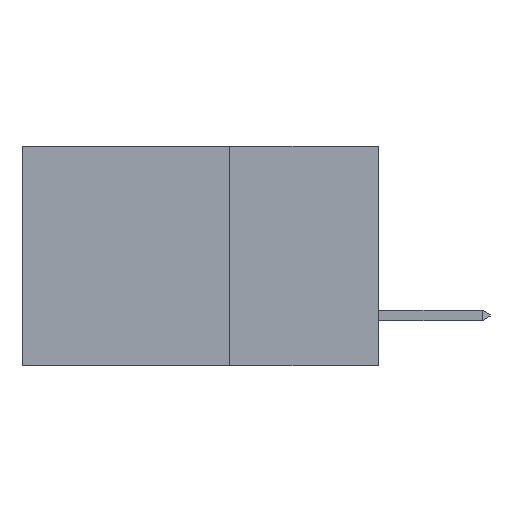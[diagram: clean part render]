
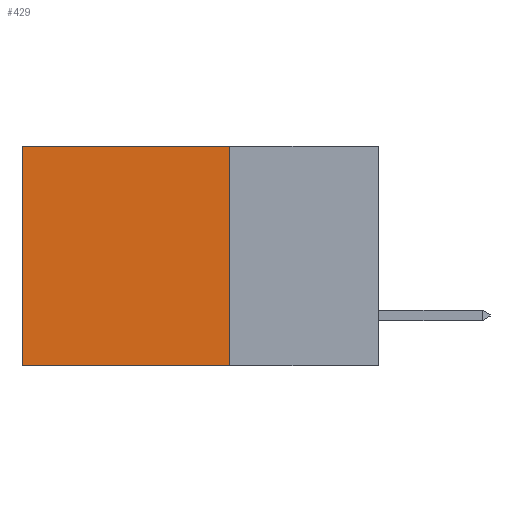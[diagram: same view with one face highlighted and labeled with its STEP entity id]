
A CAD part, left-side view. The second image highlights one B-rep face of the part: STEP entity #429.
In plain terms, the highlighted planar face has unit normal (-1, 0, 0).
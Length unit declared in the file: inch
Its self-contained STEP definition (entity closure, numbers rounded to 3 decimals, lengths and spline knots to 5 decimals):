
#268 = ORIENTED_EDGE ( 'NONE', *, *, #1162, .T. ) ;
#333 = DIRECTION ( 'NONE',  ( 0., 0., -1. ) ) ;
#345 = CARTESIAN_POINT ( 'NONE',  ( 0.2615, 0.6, -0.37 ) ) ;
#382 = CARTESIAN_POINT ( 'NONE',  ( 0.2615, 0.25, -0.37 ) ) ;
#429 = ADVANCED_FACE ( 'NONE', ( #8978 ), #9218, .F. ) ;
#729 = DIRECTION ( 'NONE',  ( 0., 0., -1. ) ) ;
#1162 = EDGE_CURVE ( 'NONE', #4390, #11350, #7078, .T. ) ;
#1446 = EDGE_CURVE ( 'NONE', #10624, #2343, #7065, .T. ) ;
#1938 = ORIENTED_EDGE ( 'NONE', *, *, #1446, .F. ) ;
#2027 = ORIENTED_EDGE ( 'NONE', *, *, #3308, .T. ) ;
#2343 = VERTEX_POINT ( 'NONE', #7645 ) ;
#2366 = LINE ( 'NONE', #345, #7023 ) ;
#3115 = DIRECTION ( 'NONE',  ( 0., 1., 0. ) ) ;
#3308 = EDGE_CURVE ( 'NONE', #11350, #2343, #2366, .T. ) ;
#4390 = VERTEX_POINT ( 'NONE', #10684 ) ;
#4483 = ORIENTED_EDGE ( 'NONE', *, *, #7222, .F. ) ;
#4650 = CARTESIAN_POINT ( 'NONE',  ( 0.2615, 0.25, -0.37 ) ) ;
#5346 = CARTESIAN_POINT ( 'NONE',  ( 0.2615, 0.25, -0.37 ) ) ;
#6020 = DIRECTION ( 'NONE',  ( 0., 0., -1. ) ) ;
#6785 = VECTOR ( 'NONE', #3115, 39.37008 ) ;
#7023 = VECTOR ( 'NONE', #333, 39.37008 ) ;
#7065 = LINE ( 'NONE', #5346, #6785 ) ;
#7078 = LINE ( 'NONE', #10170, #11368 ) ;
#7222 = EDGE_CURVE ( 'NONE', #4390, #10624, #7805, .T. ) ;
#7233 = EDGE_LOOP ( 'NONE', ( #2027, #1938, #4483, #268 ) ) ;
#7645 = CARTESIAN_POINT ( 'NONE',  ( 0.2615, 0.6, -0.37 ) ) ;
#7805 = LINE ( 'NONE', #4650, #9810 ) ;
#8076 = DIRECTION ( 'NONE',  ( 1., 0., 0. ) ) ;
#8978 = FACE_OUTER_BOUND ( 'NONE', #7233, .T. ) ;
#9218 = PLANE ( 'NONE',  #10073 ) ;
#9331 = CARTESIAN_POINT ( 'NONE',  ( 0.2615, 0.6, 0. ) ) ;
#9810 = VECTOR ( 'NONE', #729, 39.37008 ) ;
#10073 = AXIS2_PLACEMENT_3D ( 'NONE', #382, #8076, #6020 ) ;
#10170 = CARTESIAN_POINT ( 'NONE',  ( 0.2615, 0.25, 0. ) ) ;
#10269 = CARTESIAN_POINT ( 'NONE',  ( 0.2615, 0.25, -0.37 ) ) ;
#10624 = VERTEX_POINT ( 'NONE', #10269 ) ;
#10684 = CARTESIAN_POINT ( 'NONE',  ( 0.2615, 0.25, 0. ) ) ;
#11350 = VERTEX_POINT ( 'NONE', #9331 ) ;
#11368 = VECTOR ( 'NONE', #11693, 39.37008 ) ;
#11693 = DIRECTION ( 'NONE',  ( 0., 1., 0. ) ) ;
